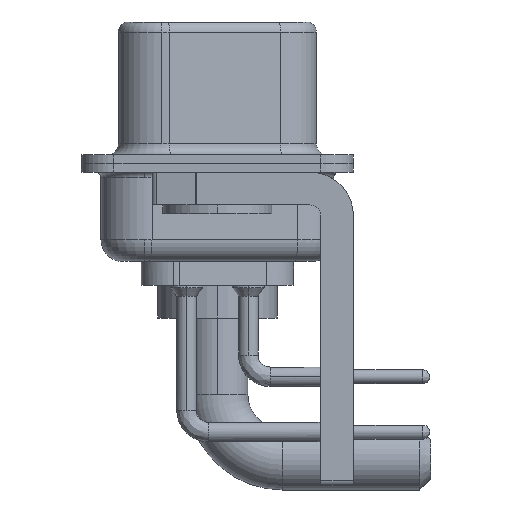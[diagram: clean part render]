
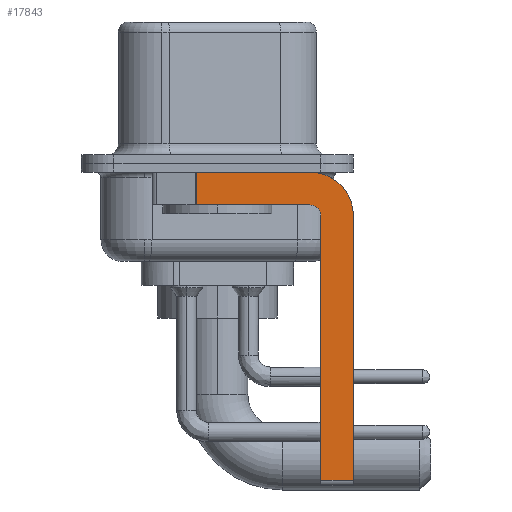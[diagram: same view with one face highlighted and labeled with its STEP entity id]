
A CAD part, left-side view. The second image highlights one B-rep face of the part: STEP entity #17843.
In plain terms, the highlighted planar face has unit normal (-1, 0, 0).
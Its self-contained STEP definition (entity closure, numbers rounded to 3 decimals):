
#379 = VERTEX_POINT ( 'NONE', #15290 ) ;
#428 = ORIENTED_EDGE ( 'NONE', *, *, #4896, .F. ) ;
#602 = DIRECTION ( 'NONE',  ( 0., 0., 1. ) ) ;
#1064 = CARTESIAN_POINT ( 'NONE',  ( -2.9, -4.75, -14.55 ) ) ;
#1807 = CARTESIAN_POINT ( 'NONE',  ( -2.9, 0.978, -1.9 ) ) ;
#2086 = CIRCLE ( 'NONE', #13461, 0.5 ) ;
#2151 = DIRECTION ( 'NONE',  ( -1., 0., 0. ) ) ;
#2157 = CARTESIAN_POINT ( 'NONE',  ( -2.9, -4.75, -2.4 ) ) ;
#2608 = CARTESIAN_POINT ( 'NONE',  ( -2.9, -6.25, -2.4 ) ) ;
#2704 = LINE ( 'NONE', #2608, #9548 ) ;
#2734 = VECTOR ( 'NONE', #17315, 1000. ) ;
#3171 = ORIENTED_EDGE ( 'NONE', *, *, #10801, .T. ) ;
#3429 = VERTEX_POINT ( 'NONE', #1807 ) ;
#3551 = DIRECTION ( 'NONE',  ( 0., 1., 0. ) ) ;
#3735 = ORIENTED_EDGE ( 'NONE', *, *, #15469, .F. ) ;
#3888 = LINE ( 'NONE', #10022, #19029 ) ;
#4030 = DIRECTION ( 'NONE',  ( 0., 0., 1. ) ) ;
#4391 = VECTOR ( 'NONE', #4030, 1000. ) ;
#4627 = ORIENTED_EDGE ( 'NONE', *, *, #20003, .F. ) ;
#4896 = EDGE_CURVE ( 'NONE', #379, #17499, #2704, .T. ) ;
#5079 = DIRECTION ( 'NONE',  ( 0., 0., -1. ) ) ;
#5384 = CIRCLE ( 'NONE', #19013, 2. ) ;
#6418 = VERTEX_POINT ( 'NONE', #1064 ) ;
#7290 = VERTEX_POINT ( 'NONE', #2157 ) ;
#7434 = CARTESIAN_POINT ( 'NONE',  ( -2.9, -4.25, -0.4 ) ) ;
#7859 = ORIENTED_EDGE ( 'NONE', *, *, #19385, .F. ) ;
#8022 = VERTEX_POINT ( 'NONE', #14101 ) ;
#9469 = DIRECTION ( 'NONE',  ( 1., 0., 0. ) ) ;
#9518 = LINE ( 'NONE', #13970, #2734 ) ;
#9548 = VECTOR ( 'NONE', #5079, 1000. ) ;
#10022 = CARTESIAN_POINT ( 'NONE',  ( -2.9, 3., -0.4 ) ) ;
#10123 = DIRECTION ( 'NONE',  ( 0., -1., 0. ) ) ;
#10610 = ORIENTED_EDGE ( 'NONE', *, *, #18895, .T. ) ;
#10801 = EDGE_CURVE ( 'NONE', #6418, #17499, #18413, .T. ) ;
#11280 = CARTESIAN_POINT ( 'NONE',  ( -2.9, -4.25, -2.4 ) ) ;
#11299 = LINE ( 'NONE', #17489, #11725 ) ;
#11374 = CARTESIAN_POINT ( 'NONE',  ( -2.9, 0.978, -0.4 ) ) ;
#11725 = VECTOR ( 'NONE', #3551, 1000. ) ;
#12512 = DIRECTION ( 'NONE',  ( 0., 0., -1. ) ) ;
#12541 = CARTESIAN_POINT ( 'NONE',  ( -2.9, -4.25, -14.55 ) ) ;
#13052 = EDGE_CURVE ( 'NONE', #8022, #3429, #11299, .T. ) ;
#13286 = VERTEX_POINT ( 'NONE', #7434 ) ;
#13334 = DIRECTION ( 'NONE',  ( 0., 0., -1. ) ) ;
#13461 = AXIS2_PLACEMENT_3D ( 'NONE', #17604, #2151, #602 ) ;
#13543 = FACE_OUTER_BOUND ( 'NONE', #18933, .T. ) ;
#13970 = CARTESIAN_POINT ( 'NONE',  ( -2.9, 0.978, -1.9 ) ) ;
#14101 = CARTESIAN_POINT ( 'NONE',  ( -2.9, -4.25, -1.9 ) ) ;
#14252 = DIRECTION ( 'NONE',  ( 0., -1., 0. ) ) ;
#14838 = LINE ( 'NONE', #17662, #4391 ) ;
#14971 = PLANE ( 'NONE',  #16163 ) ;
#15094 = VECTOR ( 'NONE', #14252, 1000. ) ;
#15290 = CARTESIAN_POINT ( 'NONE',  ( -2.9, -6.25, -2.4 ) ) ;
#15469 = EDGE_CURVE ( 'NONE', #6418, #7290, #14838, .T. ) ;
#16163 = AXIS2_PLACEMENT_3D ( 'NONE', #16686, #18205, #13334 ) ;
#16686 = CARTESIAN_POINT ( 'NONE',  ( -2.9, -4.25, -2.4 ) ) ;
#17315 = DIRECTION ( 'NONE',  ( 0., 0., -1. ) ) ;
#17489 = CARTESIAN_POINT ( 'NONE',  ( -2.9, -4.25, -1.9 ) ) ;
#17499 = VERTEX_POINT ( 'NONE', #18429 ) ;
#17569 = ORIENTED_EDGE ( 'NONE', *, *, #13052, .F. ) ;
#17604 = CARTESIAN_POINT ( 'NONE',  ( -2.9, -4.25, -2.4 ) ) ;
#17662 = CARTESIAN_POINT ( 'NONE',  ( -2.9, -4.75, -14.8 ) ) ;
#17843 = ADVANCED_FACE ( 'NONE', ( #13543 ), #14971, .F. ) ;
#18205 = DIRECTION ( 'NONE',  ( 1., 0., 0. ) ) ;
#18413 = LINE ( 'NONE', #12541, #15094 ) ;
#18429 = CARTESIAN_POINT ( 'NONE',  ( -2.9, -6.25, -14.55 ) ) ;
#18477 = ORIENTED_EDGE ( 'NONE', *, *, #19156, .F. ) ;
#18895 = EDGE_CURVE ( 'NONE', #19457, #3429, #9518, .T. ) ;
#18933 = EDGE_LOOP ( 'NONE', ( #4627, #10610, #17569, #18477, #3735, #3171, #428, #7859 ) ) ;
#19013 = AXIS2_PLACEMENT_3D ( 'NONE', #11280, #9469, #12512 ) ;
#19029 = VECTOR ( 'NONE', #10123, 1000. ) ;
#19156 = EDGE_CURVE ( 'NONE', #7290, #8022, #2086, .T. ) ;
#19385 = EDGE_CURVE ( 'NONE', #13286, #379, #5384, .T. ) ;
#19457 = VERTEX_POINT ( 'NONE', #11374 ) ;
#20003 = EDGE_CURVE ( 'NONE', #19457, #13286, #3888, .T. ) ;
